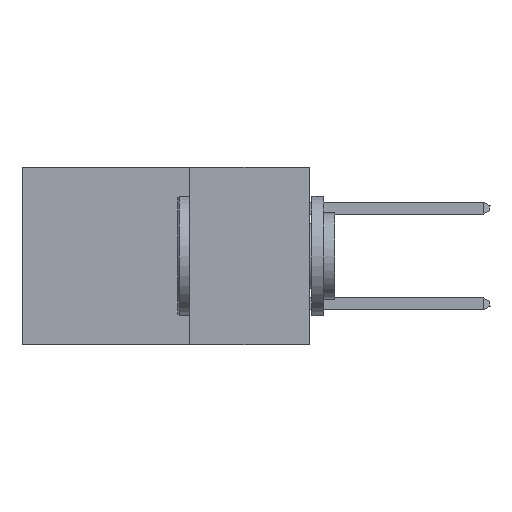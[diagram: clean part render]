
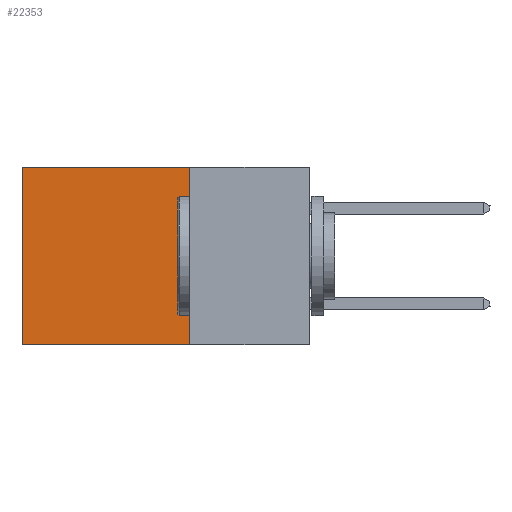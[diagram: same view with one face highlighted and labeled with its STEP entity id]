
A CAD part, left-side view. The second image highlights one B-rep face of the part: STEP entity #22353.
In plain terms, the highlighted planar face has unit normal (-1, 0, 0).
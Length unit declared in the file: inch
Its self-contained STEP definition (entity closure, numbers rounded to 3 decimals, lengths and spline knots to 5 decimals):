
#1724 = DIRECTION ( 'NONE',  ( 0., 1., 0. ) ) ;
#2851 = CARTESIAN_POINT ( 'NONE',  ( 0.2875, 0.6, 0. ) ) ;
#7444 = CARTESIAN_POINT ( 'NONE',  ( 0.2875, 0.25, 0. ) ) ;
#7822 = LINE ( 'NONE', #8722, #37784 ) ;
#8515 = VECTOR ( 'NONE', #1724, 39.37008 ) ;
#8722 = CARTESIAN_POINT ( 'NONE',  ( 0.2875, 0.25, -0.37 ) ) ;
#8834 = VECTOR ( 'NONE', #28911, 39.37008 ) ;
#10471 = ORIENTED_EDGE ( 'NONE', *, *, #33363, .T. ) ;
#10731 = DIRECTION ( 'NONE',  ( 0., 0., -1. ) ) ;
#11733 = CARTESIAN_POINT ( 'NONE',  ( 0.2875, 0.25, -0.37 ) ) ;
#13744 = EDGE_LOOP ( 'NONE', ( #38088, #26107, #17200, #10471 ) ) ;
#14930 = VERTEX_POINT ( 'NONE', #11733 ) ;
#15574 = VERTEX_POINT ( 'NONE', #2851 ) ;
#16003 = LINE ( 'NONE', #37651, #8515 ) ;
#17200 = ORIENTED_EDGE ( 'NONE', *, *, #37691, .F. ) ;
#17459 = DIRECTION ( 'NONE',  ( 0., 1., 0. ) ) ;
#17534 = CARTESIAN_POINT ( 'NONE',  ( 0.2875, 0.25, 0. ) ) ;
#18105 = VERTEX_POINT ( 'NONE', #30914 ) ;
#19584 = PLANE ( 'NONE',  #31238 ) ;
#22353 = ADVANCED_FACE ( 'NONE', ( #22725 ), #19584, .F. ) ;
#22725 = FACE_OUTER_BOUND ( 'NONE', #13744, .T. ) ;
#24759 = EDGE_CURVE ( 'NONE', #14930, #33645, #7822, .T. ) ;
#26107 = ORIENTED_EDGE ( 'NONE', *, *, #24759, .F. ) ;
#26427 = VECTOR ( 'NONE', #38509, 39.37008 ) ;
#27185 = CARTESIAN_POINT ( 'NONE',  ( 0.2875, 0.6, -0.37 ) ) ;
#28824 = EDGE_CURVE ( 'NONE', #15574, #33645, #29016, .T. ) ;
#28911 = DIRECTION ( 'NONE',  ( 0., 0., -1. ) ) ;
#29016 = LINE ( 'NONE', #31540, #8834 ) ;
#30914 = CARTESIAN_POINT ( 'NONE',  ( 0.2875, 0.25, 0. ) ) ;
#31238 = AXIS2_PLACEMENT_3D ( 'NONE', #7444, #34541, #10731 ) ;
#31540 = CARTESIAN_POINT ( 'NONE',  ( 0.2875, 0.6, 0. ) ) ;
#33363 = EDGE_CURVE ( 'NONE', #18105, #15574, #16003, .T. ) ;
#33645 = VERTEX_POINT ( 'NONE', #27185 ) ;
#34412 = LINE ( 'NONE', #17534, #26427 ) ;
#34541 = DIRECTION ( 'NONE',  ( 1., 0., 0. ) ) ;
#37651 = CARTESIAN_POINT ( 'NONE',  ( 0.2875, 0.25, 0. ) ) ;
#37691 = EDGE_CURVE ( 'NONE', #18105, #14930, #34412, .T. ) ;
#37784 = VECTOR ( 'NONE', #17459, 39.37008 ) ;
#38088 = ORIENTED_EDGE ( 'NONE', *, *, #28824, .T. ) ;
#38509 = DIRECTION ( 'NONE',  ( 0., 0., -1. ) ) ;
